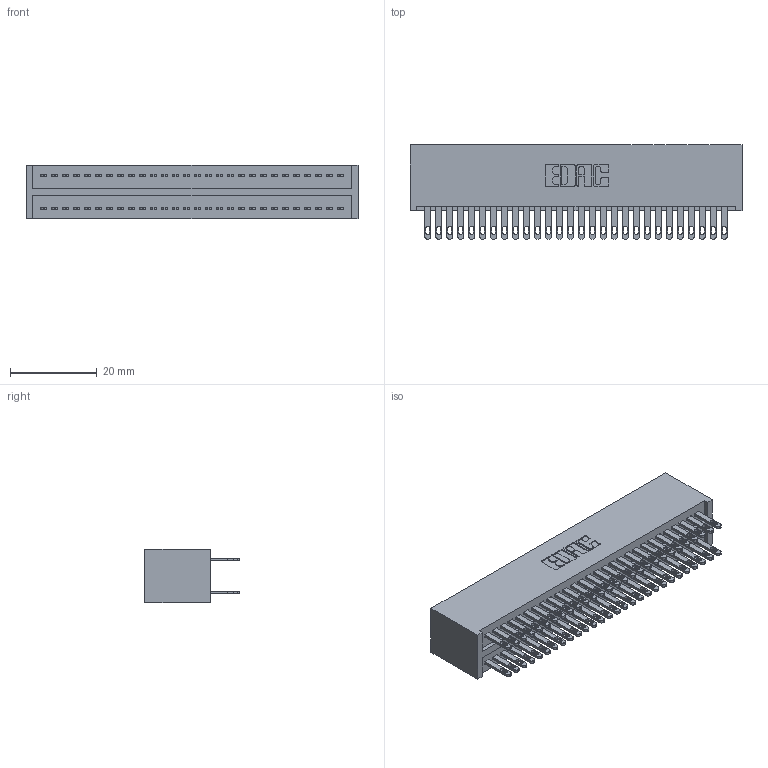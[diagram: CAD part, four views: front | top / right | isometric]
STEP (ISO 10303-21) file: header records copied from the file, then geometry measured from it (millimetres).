
FILE_DESCRIPTION (( 'STEP AP203' ), '1' );
FILE_NAME ('325-056-500-201.STEP', '2020-02-25T01:20:35', ( '' ), ( '' ), 'SwSTEP 2.0', 'SolidWorks 2016', '' );
FILE_SCHEMA (( 'CONFIG_CONTROL_DESIGN' ));
Length unit declared in the file: inch
Products named in the file (3): 325-056-500-201; 325-292-001_325-293-100; 325 Part_Lugless
Assembly tree (57 placements, depth 2):
  325-056-500-201
    325 Part_Lugless
    325-292-001_325-293-100  x56
Bounding box: 76.76 x 21.84 x 12.45 mm (x, y, z)
Volume: 10560.9 mm3; surface area: 13697.1 mm2
Topology: 57 solids, 57 shells, 2794 faces, 8519 edges, 5678 vertices
Faces by surface type: plane 1746, cylinder 1048
Entity records: 19477 total; most frequent: CARTESIAN_POINT 3242, ORIENTED_EDGE 3178, DIRECTION 2789, EDGE_CURVE 1589, VECTOR 1465, LINE 1465, VERTEX_POINT 1058, AXIS2_PLACEMENT_3D 662
